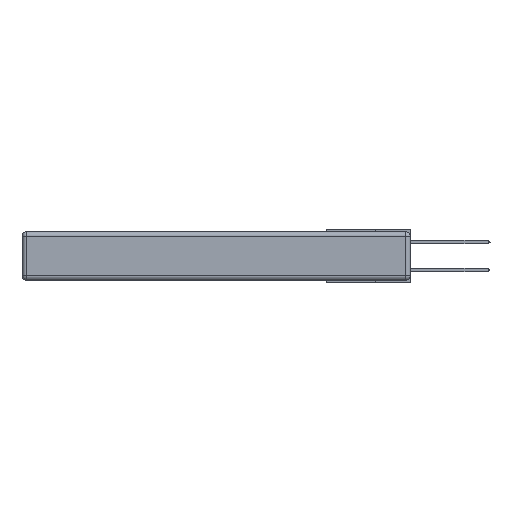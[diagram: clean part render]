
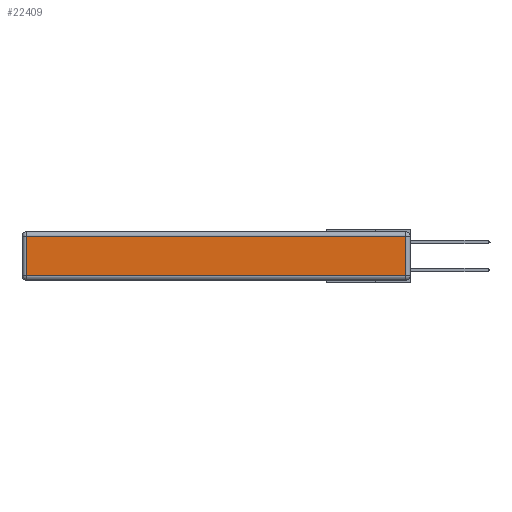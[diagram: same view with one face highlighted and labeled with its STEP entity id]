
A CAD part, left-side view. The second image highlights one B-rep face of the part: STEP entity #22409.
In plain terms, the highlighted planar face has unit normal (-1, 0, 0).
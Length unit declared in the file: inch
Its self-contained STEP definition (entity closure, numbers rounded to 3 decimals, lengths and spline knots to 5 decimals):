
#46 = AXIS2_PLACEMENT_3D ( 'NONE', #2117, #32964, #24562 ) ;
#2117 = CARTESIAN_POINT ( 'NONE',  ( 0., 0., -0.343 ) ) ;
#2768 = VECTOR ( 'NONE', #3486, 39.37008 ) ;
#3486 = DIRECTION ( 'NONE',  ( 0., 1., 0. ) ) ;
#3896 = EDGE_CURVE ( 'NONE', #22128, #30605, #28085, .T. ) ;
#4938 = LINE ( 'NONE', #19957, #2768 ) ;
#4984 = DIRECTION ( 'NONE',  ( 0., 0., -1. ) ) ;
#6329 = EDGE_CURVE ( 'NONE', #30605, #12625, #27508, .T. ) ;
#6851 = EDGE_CURVE ( 'NONE', #12625, #17086, #4938, .T. ) ;
#8118 = LINE ( 'NONE', #16242, #10728 ) ;
#8419 = CARTESIAN_POINT ( 'NONE',  ( 0., 0.03, -0.343 ) ) ;
#10728 = VECTOR ( 'NONE', #4984, 39.37008 ) ;
#11187 = ORIENTED_EDGE ( 'NONE', *, *, #3896, .T. ) ;
#12625 = VERTEX_POINT ( 'NONE', #18268 ) ;
#14052 = CARTESIAN_POINT ( 'NONE',  ( 0., 0., -0.313 ) ) ;
#16242 = CARTESIAN_POINT ( 'NONE',  ( 0., 2.72, -0.343 ) ) ;
#16918 = CARTESIAN_POINT ( 'NONE',  ( 0., 2.72, -0.313 ) ) ;
#17086 = VERTEX_POINT ( 'NONE', #21470 ) ;
#18268 = CARTESIAN_POINT ( 'NONE',  ( 0., 0.03, -0.03 ) ) ;
#18967 = PLANE ( 'NONE',  #46 ) ;
#19643 = EDGE_CURVE ( 'NONE', #17086, #22128, #8118, .T. ) ;
#19819 = ORIENTED_EDGE ( 'NONE', *, *, #6851, .T. ) ;
#19957 = CARTESIAN_POINT ( 'NONE',  ( 0., 2.75, -0.03 ) ) ;
#21312 = ORIENTED_EDGE ( 'NONE', *, *, #19643, .T. ) ;
#21470 = CARTESIAN_POINT ( 'NONE',  ( 0., 2.72, -0.03 ) ) ;
#21598 = ORIENTED_EDGE ( 'NONE', *, *, #6329, .T. ) ;
#22128 = VERTEX_POINT ( 'NONE', #16918 ) ;
#22409 = ADVANCED_FACE ( 'NONE', ( #22612 ), #18967, .T. ) ;
#22612 = FACE_OUTER_BOUND ( 'NONE', #25463, .T. ) ;
#24562 = DIRECTION ( 'NONE',  ( 0., 0., 1. ) ) ;
#25463 = EDGE_LOOP ( 'NONE', ( #11187, #21598, #19819, #21312 ) ) ;
#27508 = LINE ( 'NONE', #8419, #29248 ) ;
#28085 = LINE ( 'NONE', #14052, #30271 ) ;
#29248 = VECTOR ( 'NONE', #29470, 39.37008 ) ;
#29470 = DIRECTION ( 'NONE',  ( 0., 0., 1. ) ) ;
#30271 = VECTOR ( 'NONE', #33602, 39.37008 ) ;
#30407 = CARTESIAN_POINT ( 'NONE',  ( 0., 0.03, -0.313 ) ) ;
#30605 = VERTEX_POINT ( 'NONE', #30407 ) ;
#32964 = DIRECTION ( 'NONE',  ( -1., 0., 0. ) ) ;
#33602 = DIRECTION ( 'NONE',  ( 0., -1., 0. ) ) ;
